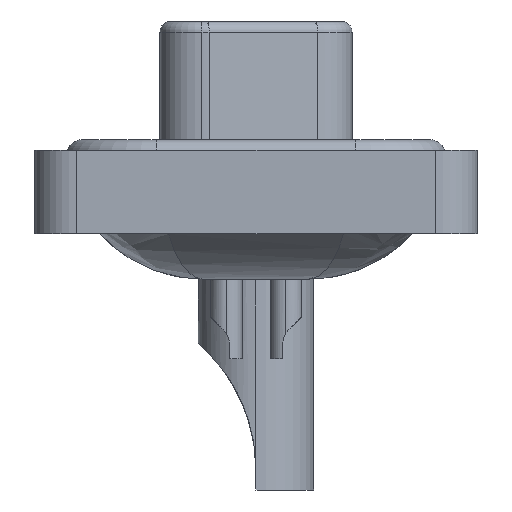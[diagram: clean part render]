
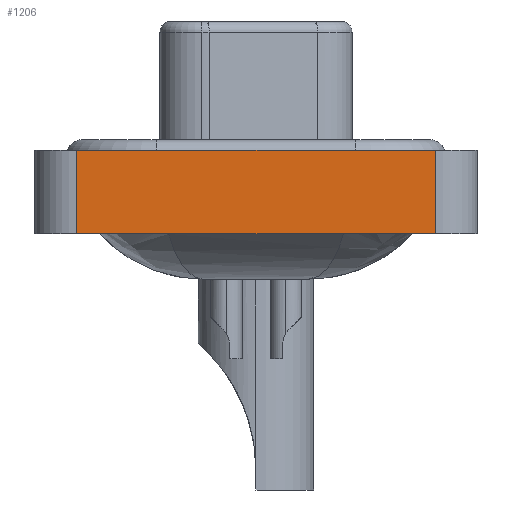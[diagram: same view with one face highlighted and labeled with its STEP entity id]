
A CAD part, left-side view. The second image highlights one B-rep face of the part: STEP entity #1206.
In plain terms, the highlighted planar face has unit normal (-1, 0, 0).
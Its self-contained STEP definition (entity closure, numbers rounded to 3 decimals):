
#1206 = ADVANCED_FACE ( 'NONE', ( #5433 ), #5946, .T. ) ;
#1671 = DIRECTION ( 'NONE',  ( 0., 0., 1. ) ) ;
#1708 = AXIS2_PLACEMENT_3D ( 'NONE', #13054, #11559, #1671 ) ;
#2917 = ORIENTED_EDGE ( 'NONE', *, *, #4658, .F. ) ;
#3476 = DIRECTION ( 'NONE',  ( 0., -1., 0. ) ) ;
#3591 = CARTESIAN_POINT ( 'NONE',  ( -7.35, -8.55, 0.4 ) ) ;
#3603 = DIRECTION ( 'NONE',  ( 0., -1., 0. ) ) ;
#4022 = EDGE_CURVE ( 'NONE', #13210, #6336, #16749, .T. ) ;
#4658 = EDGE_CURVE ( 'NONE', #13210, #5364, #11087, .T. ) ;
#5121 = CARTESIAN_POINT ( 'NONE',  ( -7.35, -8.55, -3.6 ) ) ;
#5364 = VERTEX_POINT ( 'NONE', #14637 ) ;
#5433 = FACE_OUTER_BOUND ( 'NONE', #18351, .T. ) ;
#5946 = PLANE ( 'NONE',  #1708 ) ;
#6336 = VERTEX_POINT ( 'NONE', #8046 ) ;
#6532 = VERTEX_POINT ( 'NONE', #8678 ) ;
#7222 = CARTESIAN_POINT ( 'NONE',  ( -7.35, 8.55, -3.6 ) ) ;
#8046 = CARTESIAN_POINT ( 'NONE',  ( -7.35, -8.55, -3.6 ) ) ;
#8652 = CARTESIAN_POINT ( 'NONE',  ( -7.35, -8.55, -3.6 ) ) ;
#8678 = CARTESIAN_POINT ( 'NONE',  ( -7.35, -8.55, 0.4 ) ) ;
#10388 = LINE ( 'NONE', #8652, #10939 ) ;
#10939 = VECTOR ( 'NONE', #23414, 1000. ) ;
#10953 = CARTESIAN_POINT ( 'NONE',  ( -7.35, 8.55, -3.6 ) ) ;
#11087 = LINE ( 'NONE', #7222, #16685 ) ;
#11559 = DIRECTION ( 'NONE',  ( -1., 0., 0. ) ) ;
#13054 = CARTESIAN_POINT ( 'NONE',  ( -7.35, -8.55, -3.6 ) ) ;
#13210 = VERTEX_POINT ( 'NONE', #10953 ) ;
#14637 = CARTESIAN_POINT ( 'NONE',  ( -7.35, 8.55, 0.4 ) ) ;
#14838 = DIRECTION ( 'NONE',  ( 0., 0., 1. ) ) ;
#16685 = VECTOR ( 'NONE', #14838, 1000. ) ;
#16749 = LINE ( 'NONE', #5121, #19059 ) ;
#18351 = EDGE_LOOP ( 'NONE', ( #20073, #23474, #2917, #23506 ) ) ;
#19059 = VECTOR ( 'NONE', #3603, 1000. ) ;
#19331 = VECTOR ( 'NONE', #3476, 1000. ) ;
#20073 = ORIENTED_EDGE ( 'NONE', *, *, #22300, .T. ) ;
#20738 = LINE ( 'NONE', #3591, #19331 ) ;
#22300 = EDGE_CURVE ( 'NONE', #6336, #6532, #10388, .T. ) ;
#23009 = EDGE_CURVE ( 'NONE', #5364, #6532, #20738, .T. ) ;
#23414 = DIRECTION ( 'NONE',  ( 0., 0., 1. ) ) ;
#23474 = ORIENTED_EDGE ( 'NONE', *, *, #23009, .F. ) ;
#23506 = ORIENTED_EDGE ( 'NONE', *, *, #4022, .T. ) ;
